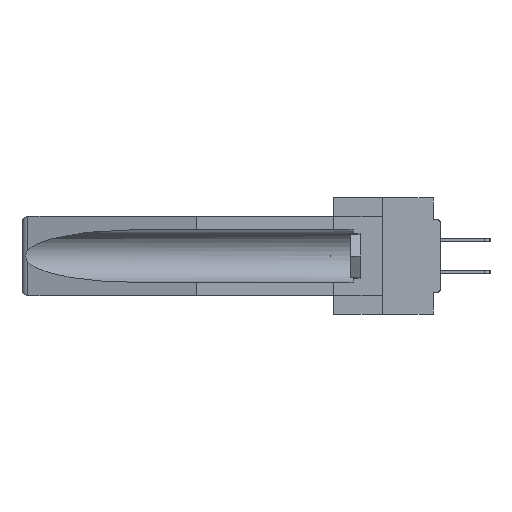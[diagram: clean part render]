
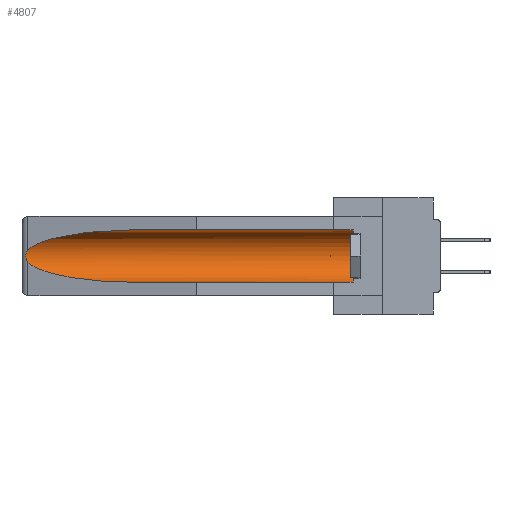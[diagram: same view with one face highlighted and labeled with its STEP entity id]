
A CAD part, left-side view. The second image highlights one B-rep face of the part: STEP entity #4807.
In plain terms, the highlighted cylindrical face has radius 2.857 mm (diameter 5.715 mm), a partial arc.
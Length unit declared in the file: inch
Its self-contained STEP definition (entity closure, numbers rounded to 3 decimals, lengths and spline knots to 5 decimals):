
#651 = AXIS2_PLACEMENT_3D ( 'NONE', #31534, #19997, #27973 ) ;
#896 = CARTESIAN_POINT ( 'NONE',  ( 0.26537, 1.52718, -0.14972 ) ) ;
#1532 = CARTESIAN_POINT ( 'NONE',  ( 0.2673, 1.53269, -0.17917 ) ) ;
#1610 = VECTOR ( 'NONE', #6560, 39.37008 ) ;
#1710 = CARTESIAN_POINT ( 'NONE',  ( 0.155, 1.07973, -0.059 ) ) ;
#2772 = DIRECTION ( 'NONE',  ( 0., 0., 1. ) ) ;
#2827 = ORIENTED_EDGE ( 'NONE', *, *, #36608, .T. ) ;
#4243 = CYLINDRICAL_SURFACE ( 'NONE', #42239, 0.1125 ) ;
#4623 = CARTESIAN_POINT ( 'NONE',  ( 0.26537, 1.52718, -0.19328 ) ) ;
#4807 = ADVANCED_FACE ( 'NONE', ( #15181 ), #4243, .F. ) ;
#5759 = CARTESIAN_POINT ( 'NONE',  ( 0.155, -0.30754, -0.284 ) ) ;
#6560 = DIRECTION ( 'NONE',  ( 0., 1., 0. ) ) ;
#6666 = ORIENTED_EDGE ( 'NONE', *, *, #29046, .T. ) ;
#8645 = CARTESIAN_POINT ( 'NONE',  ( 0.155, 1.07973, -0.284 ) ) ;
#8934 = VERTEX_POINT ( 'NONE', #8645 ) ;
#11866 = CARTESIAN_POINT ( 'NONE',  ( 0.26654, 1.53092, -0.15636 ) ) ;
#12509 = CARTESIAN_POINT ( 'NONE',  ( 0.26597, 1.52961, -0.15275 ) ) ;
#15181 = FACE_OUTER_BOUND ( 'NONE', #19357, .T. ) ;
#15563 = CARTESIAN_POINT ( 'NONE',  ( 0.2673, 1.5327, -0.16383 ) ) ;
#18742 = CARTESIAN_POINT ( 'NONE',  ( 0.155, 1.07973, -0.284 ) ) ;
#18981 = EDGE_CURVE ( 'NONE', #46913, #8934, #20760, .T. ) ;
#19357 = EDGE_LOOP ( 'NONE', ( #2827, #40938, #6666, #45231, #37366, #41180 ) ) ;
#19997 = DIRECTION ( 'NONE',  ( 0., -1., 0. ) ) ;
#20062 = CARTESIAN_POINT ( 'NONE',  ( 0.26537, 1.52718, -0.19328 ) ) ;
#20550 = DIRECTION ( 'NONE',  ( 0., 1., 0. ) ) ;
#20581 = B_SPLINE_CURVE_WITH_KNOTS ( 'NONE', 3,
 ( #896, #12509, #11866, #15563, #26596, #45377, #1532, #23219, #41286, #4623 ),
 .UNSPECIFIED., .F., .F.,
 ( 4, 2, 2, 2, 4 ),
 ( 0., 0.00029, 0.00058, 0.00087, 0.00117 ),
 .UNSPECIFIED. ) ;
#20760 = LINE ( 'NONE', #5759, #31681 ) ;
#21155 =( BOUNDED_CURVE ( )  B_SPLINE_CURVE ( 3, ( #1710, #45878, #30939, #34668 ),
 .UNSPECIFIED., .F., .F. ) 
 B_SPLINE_CURVE_WITH_KNOTS ( ( 4, 4 ),
 ( 4.71239, 6.08839 ),
 .UNSPECIFIED. ) 
 CURVE ( )  GEOMETRIC_REPRESENTATION_ITEM ( )  RATIONAL_B_SPLINE_CURVE ( ( 1., 0.848, 0.848, 1. ) ) 
 REPRESENTATION_ITEM ( '' )  );
#21463 = VERTEX_POINT ( 'NONE', #38544 ) ;
#22045 = EDGE_CURVE ( 'NONE', #46913, #26792, #47489, .T. ) ;
#23219 = CARTESIAN_POINT ( 'NONE',  ( 0.26655, 1.53094, -0.18657 ) ) ;
#23236 = CARTESIAN_POINT ( 'NONE',  ( 0.155, -0.30754, -0.1715 ) ) ;
#23393 = DIRECTION ( 'NONE',  ( 0., 1., 0. ) ) ;
#26596 = CARTESIAN_POINT ( 'NONE',  ( 0.2675, 1.53308, -0.16763 ) ) ;
#26680 = CARTESIAN_POINT ( 'NONE',  ( 0.26537, 1.52718, -0.14972 ) ) ;
#26792 = VERTEX_POINT ( 'NONE', #46253 ) ;
#27973 = DIRECTION ( 'NONE',  ( 0., 0., 1. ) ) ;
#28977 = CARTESIAN_POINT ( 'NONE',  ( 0.21114, 1.30732, -0.284 ) ) ;
#29046 = EDGE_CURVE ( 'NONE', #32849, #8934, #36181, .T. ) ;
#30939 = CARTESIAN_POINT ( 'NONE',  ( 0.25451, 1.48313, -0.09465 ) ) ;
#31534 = CARTESIAN_POINT ( 'NONE',  ( 0.155, 0.126, -0.1715 ) ) ;
#31681 = VECTOR ( 'NONE', #20550, 39.37008 ) ;
#32394 = CARTESIAN_POINT ( 'NONE',  ( 0.25451, 1.48313, -0.24835 ) ) ;
#32849 = VERTEX_POINT ( 'NONE', #20062 ) ;
#33828 = EDGE_CURVE ( 'NONE', #46102, #32849, #20581, .T. ) ;
#34668 = CARTESIAN_POINT ( 'NONE',  ( 0.26537, 1.52718, -0.14972 ) ) ;
#36181 =( BOUNDED_CURVE ( )  B_SPLINE_CURVE ( 3, ( #47514, #32394, #28977, #18742 ),
 .UNSPECIFIED., .F., .F. ) 
 B_SPLINE_CURVE_WITH_KNOTS ( ( 4, 4 ),
 ( 0.1948, 1.5708 ),
 .UNSPECIFIED. ) 
 CURVE ( )  GEOMETRIC_REPRESENTATION_ITEM ( )  RATIONAL_B_SPLINE_CURVE ( ( 1., 0.848, 0.848, 1. ) ) 
 REPRESENTATION_ITEM ( '' )  );
#36608 = EDGE_CURVE ( 'NONE', #21463, #46102, #21155, .T. ) ;
#36785 = EDGE_CURVE ( 'NONE', #26792, #21463, #43086, .T. ) ;
#37366 = ORIENTED_EDGE ( 'NONE', *, *, #22045, .T. ) ;
#37688 = CARTESIAN_POINT ( 'NONE',  ( 0.155, 0.126, -0.284 ) ) ;
#38544 = CARTESIAN_POINT ( 'NONE',  ( 0.155, 1.07973, -0.059 ) ) ;
#39494 = CARTESIAN_POINT ( 'NONE',  ( 0.155, -0.30754, -0.059 ) ) ;
#40938 = ORIENTED_EDGE ( 'NONE', *, *, #33828, .T. ) ;
#41180 = ORIENTED_EDGE ( 'NONE', *, *, #36785, .T. ) ;
#41286 = CARTESIAN_POINT ( 'NONE',  ( 0.26597, 1.5296, -0.19026 ) ) ;
#42239 = AXIS2_PLACEMENT_3D ( 'NONE', #23236, #23393, #2772 ) ;
#43086 = LINE ( 'NONE', #39494, #1610 ) ;
#45231 = ORIENTED_EDGE ( 'NONE', *, *, #18981, .F. ) ;
#45377 = CARTESIAN_POINT ( 'NONE',  ( 0.2675, 1.53308, -0.17534 ) ) ;
#45878 = CARTESIAN_POINT ( 'NONE',  ( 0.21114, 1.30732, -0.059 ) ) ;
#46102 = VERTEX_POINT ( 'NONE', #26680 ) ;
#46253 = CARTESIAN_POINT ( 'NONE',  ( 0.155, 0.126, -0.059 ) ) ;
#46913 = VERTEX_POINT ( 'NONE', #37688 ) ;
#47489 = CIRCLE ( 'NONE', #651, 0.1125 ) ;
#47514 = CARTESIAN_POINT ( 'NONE',  ( 0.26537, 1.52718, -0.19328 ) ) ;
